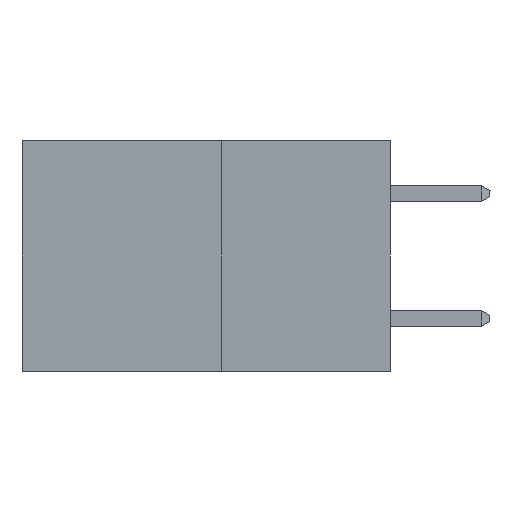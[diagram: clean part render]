
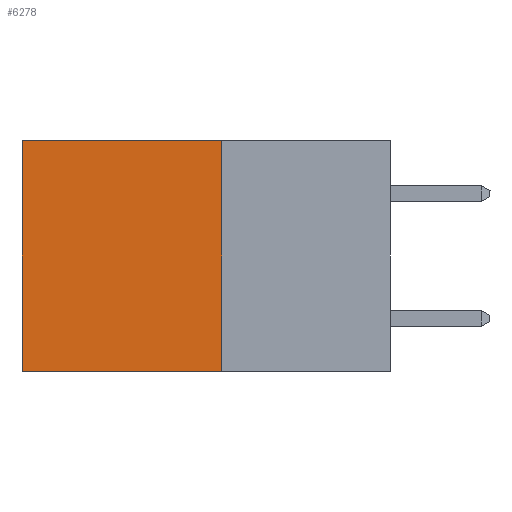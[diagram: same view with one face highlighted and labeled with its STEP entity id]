
A CAD part, left-side view. The second image highlights one B-rep face of the part: STEP entity #6278.
In plain terms, the highlighted planar face has unit normal (-1, 0, 0).
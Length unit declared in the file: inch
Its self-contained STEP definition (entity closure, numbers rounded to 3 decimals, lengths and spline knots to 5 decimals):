
#95 = LINE ( 'NONE', #5969, #6769 ) ;
#645 = EDGE_CURVE ( 'NONE', #7248, #3065, #6695, .T. ) ;
#988 = EDGE_LOOP ( 'NONE', ( #1138, #4392, #4395, #4353 ) ) ;
#1138 = ORIENTED_EDGE ( 'NONE', *, *, #3855, .T. ) ;
#1422 = VECTOR ( 'NONE', #8322, 39.37008 ) ;
#1597 = LINE ( 'NONE', #7805, #1871 ) ;
#1871 = VECTOR ( 'NONE', #5456, 39.37008 ) ;
#2383 = VERTEX_POINT ( 'NONE', #5330 ) ;
#2682 = CARTESIAN_POINT ( 'NONE',  ( 0.277, 0.59, 0. ) ) ;
#2882 = DIRECTION ( 'NONE',  ( 1., 0., 0. ) ) ;
#3065 = VERTEX_POINT ( 'NONE', #7710 ) ;
#3787 = EDGE_CURVE ( 'NONE', #7248, #4771, #95, .T. ) ;
#3855 = EDGE_CURVE ( 'NONE', #4771, #2383, #8011, .T. ) ;
#4353 = ORIENTED_EDGE ( 'NONE', *, *, #3787, .T. ) ;
#4392 = ORIENTED_EDGE ( 'NONE', *, *, #8301, .F. ) ;
#4395 = ORIENTED_EDGE ( 'NONE', *, *, #645, .F. ) ;
#4396 = VECTOR ( 'NONE', #7329, 39.37008 ) ;
#4771 = VERTEX_POINT ( 'NONE', #2682 ) ;
#5075 = DIRECTION ( 'NONE',  ( 0., 1., 0. ) ) ;
#5308 = CARTESIAN_POINT ( 'NONE',  ( 0.277, 0.27, -0.37 ) ) ;
#5330 = CARTESIAN_POINT ( 'NONE',  ( 0.277, 0.59, -0.37 ) ) ;
#5456 = DIRECTION ( 'NONE',  ( 0., 1., 0. ) ) ;
#5969 = CARTESIAN_POINT ( 'NONE',  ( 0.277, 0.27, 0. ) ) ;
#6262 = CARTESIAN_POINT ( 'NONE',  ( 0.277, 0.27, -0.37 ) ) ;
#6278 = ADVANCED_FACE ( 'NONE', ( #9070 ), #8403, .F. ) ;
#6695 = LINE ( 'NONE', #6262, #4396 ) ;
#6769 = VECTOR ( 'NONE', #5075, 39.37008 ) ;
#7248 = VERTEX_POINT ( 'NONE', #10426 ) ;
#7329 = DIRECTION ( 'NONE',  ( 0., 0., -1. ) ) ;
#7610 = CARTESIAN_POINT ( 'NONE',  ( 0.277, 0.59, -0.37 ) ) ;
#7710 = CARTESIAN_POINT ( 'NONE',  ( 0.277, 0.27, -0.37 ) ) ;
#7805 = CARTESIAN_POINT ( 'NONE',  ( 0.277, 0.27, -0.37 ) ) ;
#8011 = LINE ( 'NONE', #7610, #1422 ) ;
#8301 = EDGE_CURVE ( 'NONE', #3065, #2383, #1597, .T. ) ;
#8322 = DIRECTION ( 'NONE',  ( 0., 0., -1. ) ) ;
#8403 = PLANE ( 'NONE',  #9278 ) ;
#8444 = DIRECTION ( 'NONE',  ( 0., 0., -1. ) ) ;
#9070 = FACE_OUTER_BOUND ( 'NONE', #988, .T. ) ;
#9278 = AXIS2_PLACEMENT_3D ( 'NONE', #5308, #2882, #8444 ) ;
#10426 = CARTESIAN_POINT ( 'NONE',  ( 0.277, 0.27, 0. ) ) ;
